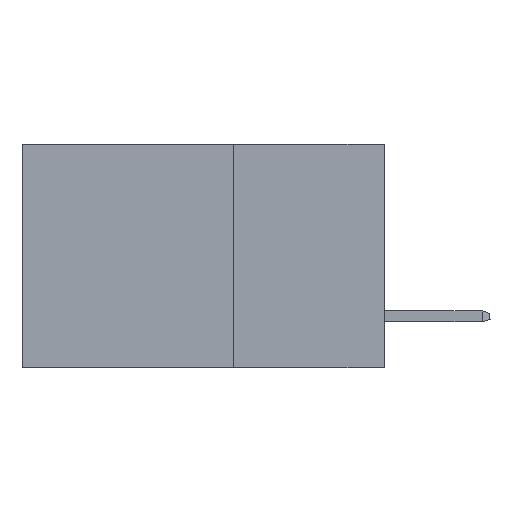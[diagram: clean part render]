
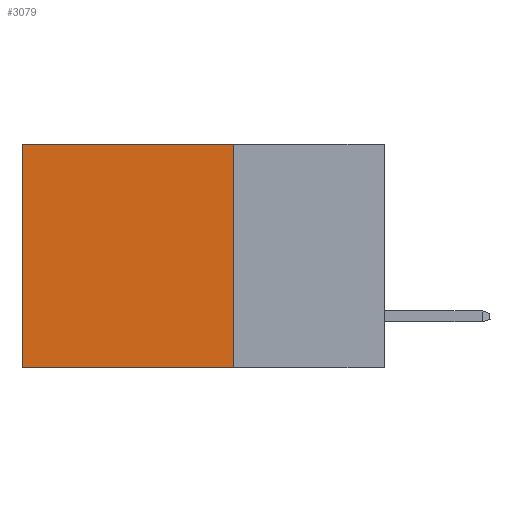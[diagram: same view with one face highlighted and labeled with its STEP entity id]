
A CAD part, left-side view. The second image highlights one B-rep face of the part: STEP entity #3079.
In plain terms, the highlighted planar face has unit normal (-1, 0, 0).
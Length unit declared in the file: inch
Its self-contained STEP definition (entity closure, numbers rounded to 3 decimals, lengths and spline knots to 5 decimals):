
#93 = AXIS2_PLACEMENT_3D ( 'NONE', #13938, #3699, #6436 ) ;
#378 = DIRECTION ( 'NONE',  ( 0., 0., -1. ) ) ;
#787 = VECTOR ( 'NONE', #378, 39.37008 ) ;
#1502 = LINE ( 'NONE', #13412, #10482 ) ;
#1630 = CARTESIAN_POINT ( 'NONE',  ( 0.298, 0.25, 0. ) ) ;
#1803 = FACE_OUTER_BOUND ( 'NONE', #13144, .T. ) ;
#1956 = VERTEX_POINT ( 'NONE', #6734 ) ;
#2737 = VERTEX_POINT ( 'NONE', #10774 ) ;
#3079 = ADVANCED_FACE ( 'NONE', ( #1803 ), #16262, .F. ) ;
#3584 = DIRECTION ( 'NONE',  ( 0., 1., 0. ) ) ;
#3699 = DIRECTION ( 'NONE',  ( 1., 0., 0. ) ) ;
#4334 = CARTESIAN_POINT ( 'NONE',  ( 0.298, 0.6, 0. ) ) ;
#4553 = EDGE_CURVE ( 'NONE', #15907, #7611, #5705, .T. ) ;
#5583 = LINE ( 'NONE', #1630, #787 ) ;
#5705 = LINE ( 'NONE', #4334, #8291 ) ;
#5785 = DIRECTION ( 'NONE',  ( 0., 1., 0. ) ) ;
#6161 = CARTESIAN_POINT ( 'NONE',  ( 0.298, 0.6, 0. ) ) ;
#6436 = DIRECTION ( 'NONE',  ( 0., 0., -1. ) ) ;
#6734 = CARTESIAN_POINT ( 'NONE',  ( 0.298, 0.25, -0.37 ) ) ;
#7611 = VERTEX_POINT ( 'NONE', #10095 ) ;
#7745 = ORIENTED_EDGE ( 'NONE', *, *, #13261, .F. ) ;
#8125 = EDGE_CURVE ( 'NONE', #1956, #7611, #11440, .T. ) ;
#8170 = DIRECTION ( 'NONE',  ( 0., 0., -1. ) ) ;
#8291 = VECTOR ( 'NONE', #8170, 39.37008 ) ;
#9964 = CARTESIAN_POINT ( 'NONE',  ( 0.298, 0.25, -0.37 ) ) ;
#10095 = CARTESIAN_POINT ( 'NONE',  ( 0.298, 0.6, -0.37 ) ) ;
#10482 = VECTOR ( 'NONE', #5785, 39.37008 ) ;
#10774 = CARTESIAN_POINT ( 'NONE',  ( 0.298, 0.25, 0. ) ) ;
#11440 = LINE ( 'NONE', #9964, #12410 ) ;
#12172 = ORIENTED_EDGE ( 'NONE', *, *, #16107, .T. ) ;
#12410 = VECTOR ( 'NONE', #3584, 39.37008 ) ;
#13144 = EDGE_LOOP ( 'NONE', ( #15865, #16116, #7745, #12172 ) ) ;
#13261 = EDGE_CURVE ( 'NONE', #2737, #1956, #5583, .T. ) ;
#13412 = CARTESIAN_POINT ( 'NONE',  ( 0.298, 0.25, 0. ) ) ;
#13938 = CARTESIAN_POINT ( 'NONE',  ( 0.298, 0.25, 0. ) ) ;
#15865 = ORIENTED_EDGE ( 'NONE', *, *, #4553, .T. ) ;
#15907 = VERTEX_POINT ( 'NONE', #6161 ) ;
#16107 = EDGE_CURVE ( 'NONE', #2737, #15907, #1502, .T. ) ;
#16116 = ORIENTED_EDGE ( 'NONE', *, *, #8125, .F. ) ;
#16262 = PLANE ( 'NONE',  #93 ) ;
